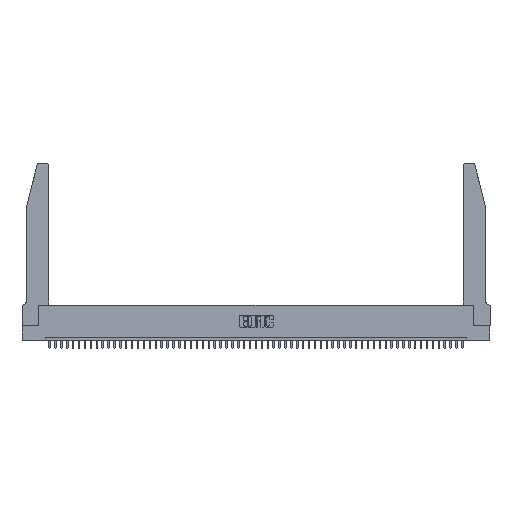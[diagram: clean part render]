
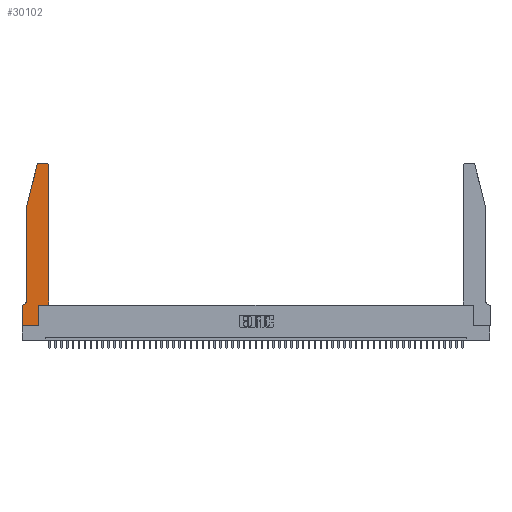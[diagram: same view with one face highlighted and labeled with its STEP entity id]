
A CAD part, top view. The second image highlights one B-rep face of the part: STEP entity #30102.
In plain terms, the highlighted planar face has unit normal (0, 0, 1).
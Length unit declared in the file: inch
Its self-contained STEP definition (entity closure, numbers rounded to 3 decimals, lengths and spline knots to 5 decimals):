
#16 = ORIENTED_EDGE ( 'NONE', *, *, #2910, .T. ) ;
#174 = VERTEX_POINT ( 'NONE', #38158 ) ;
#950 = CIRCLE ( 'NONE', #13804, 0.03 ) ;
#1086 = ORIENTED_EDGE ( 'NONE', *, *, #50567, .T. ) ;
#1452 = CARTESIAN_POINT ( 'NONE',  ( 0.0755, 0.42, 0.37 ) ) ;
#2910 = EDGE_CURVE ( 'NONE', #40060, #28558, #23130, .T. ) ;
#2999 = DIRECTION ( 'NONE',  ( -1., 0., 0. ) ) ;
#3497 = DIRECTION ( 'NONE',  ( -0.239, -0.971, 0. ) ) ;
#4057 = CARTESIAN_POINT ( 'NONE',  ( 0.0755, 2., 0.37 ) ) ;
#4463 = LINE ( 'NONE', #9818, #31969 ) ;
#4713 = CARTESIAN_POINT ( 'NONE',  ( 0.25487, 2.72718, 0.37 ) ) ;
#5218 = CARTESIAN_POINT ( 'NONE',  ( 0.2865, 0.35, 0.37 ) ) ;
#5558 = EDGE_CURVE ( 'NONE', #18067, #16991, #46507, .T. ) ;
#5904 = LINE ( 'NONE', #52612, #53746 ) ;
#6494 = EDGE_CURVE ( 'NONE', #16991, #28098, #20260, .T. ) ;
#6971 = CARTESIAN_POINT ( 'NONE',  ( 0.0755, 0.35, 0.37 ) ) ;
#7023 = CARTESIAN_POINT ( 'NONE',  ( 0.284, 2.72, 0.37 ) ) ;
#7077 = DIRECTION ( 'NONE',  ( 1., 0., 0. ) ) ;
#8402 = CARTESIAN_POINT ( 'NONE',  ( 0., 0., 0.37 ) ) ;
#9818 = CARTESIAN_POINT ( 'NONE',  ( 0., 0., 0.37 ) ) ;
#10351 = CARTESIAN_POINT ( 'NONE',  ( 0.0755, 2., 0.37 ) ) ;
#11780 = VECTOR ( 'NONE', #2999, 39.37008 ) ;
#13215 = ORIENTED_EDGE ( 'NONE', *, *, #16673, .T. ) ;
#13804 = AXIS2_PLACEMENT_3D ( 'NONE', #43182, #18163, #30705 ) ;
#14008 = CARTESIAN_POINT ( 'NONE',  ( 0.284, 2.75, 0.37 ) ) ;
#14403 = ORIENTED_EDGE ( 'NONE', *, *, #17126, .T. ) ;
#14758 = CARTESIAN_POINT ( 'NONE',  ( 0.2865, 0.35, 0.37 ) ) ;
#15021 = DIRECTION ( 'NONE',  ( 0., 0., 1. ) ) ;
#15152 = DIRECTION ( 'NONE',  ( 0., 1., 0. ) ) ;
#15255 = CIRCLE ( 'NONE', #50431, 0.03 ) ;
#15518 = ORIENTED_EDGE ( 'NONE', *, *, #6494, .T. ) ;
#15638 = LINE ( 'NONE', #10351, #32529 ) ;
#15873 = ORIENTED_EDGE ( 'NONE', *, *, #5558, .T. ) ;
#16673 = EDGE_CURVE ( 'NONE', #34504, #174, #27678, .T. ) ;
#16991 = VERTEX_POINT ( 'NONE', #47603 ) ;
#17126 = EDGE_CURVE ( 'NONE', #28558, #34760, #4463, .T. ) ;
#17492 = ORIENTED_EDGE ( 'NONE', *, *, #36888, .T. ) ;
#17604 = VERTEX_POINT ( 'NONE', #51350 ) ;
#17742 = VERTEX_POINT ( 'NONE', #1452 ) ;
#17842 = CARTESIAN_POINT ( 'NONE',  ( 0., 0.35, 0.37 ) ) ;
#18067 = VERTEX_POINT ( 'NONE', #5218 ) ;
#18163 = DIRECTION ( 'NONE',  ( 0., 0., 1. ) ) ;
#19186 = FACE_OUTER_BOUND ( 'NONE', #41227, .T. ) ;
#20111 = DIRECTION ( 'NONE',  ( -1., 0., 0. ) ) ;
#20260 = LINE ( 'NONE', #21286, #35879 ) ;
#20786 = VERTEX_POINT ( 'NONE', #26164 ) ;
#21286 = CARTESIAN_POINT ( 'NONE',  ( 0.4505, 0.35, 0.37 ) ) ;
#23130 = LINE ( 'NONE', #6971, #32956 ) ;
#23139 = DIRECTION ( 'NONE',  ( 0., -1., 0. ) ) ;
#23240 = DIRECTION ( 'NONE',  ( 1., 0., 0. ) ) ;
#25009 = EDGE_CURVE ( 'NONE', #28098, #20786, #950, .T. ) ;
#25452 = LINE ( 'NONE', #44605, #11780 ) ;
#26164 = CARTESIAN_POINT ( 'NONE',  ( 0.4205, 2.75, 0.37 ) ) ;
#26888 = AXIS2_PLACEMENT_3D ( 'NONE', #52086, #15021, #40216 ) ;
#26950 = EDGE_CURVE ( 'NONE', #17742, #40060, #48659, .T. ) ;
#27076 = ORIENTED_EDGE ( 'NONE', *, *, #30351, .T. ) ;
#27678 = LINE ( 'NONE', #4057, #43295 ) ;
#27837 = DIRECTION ( 'NONE',  ( 1., 0., 0. ) ) ;
#28098 = VERTEX_POINT ( 'NONE', #28202 ) ;
#28202 = CARTESIAN_POINT ( 'NONE',  ( 0.4505, 2.72, 0.37 ) ) ;
#28558 = VERTEX_POINT ( 'NONE', #17842 ) ;
#30102 = ADVANCED_FACE ( 'NONE', ( #19186 ), #40026, .T. ) ;
#30351 = EDGE_CURVE ( 'NONE', #46206, #34504, #15255, .T. ) ;
#30705 = DIRECTION ( 'NONE',  ( 1., 0., 0. ) ) ;
#31969 = VECTOR ( 'NONE', #23139, 39.37008 ) ;
#32529 = VECTOR ( 'NONE', #52026, 39.37008 ) ;
#32691 = EDGE_CURVE ( 'NONE', #20786, #46206, #25452, .T. ) ;
#32853 = CARTESIAN_POINT ( 'NONE',  ( 0.0055, 0.35, 0.37 ) ) ;
#32956 = VECTOR ( 'NONE', #40247, 39.37008 ) ;
#34504 = VERTEX_POINT ( 'NONE', #4713 ) ;
#34760 = VERTEX_POINT ( 'NONE', #8402 ) ;
#35879 = VECTOR ( 'NONE', #50223, 39.37008 ) ;
#36888 = EDGE_CURVE ( 'NONE', #34760, #17604, #5904, .T. ) ;
#37429 = ORIENTED_EDGE ( 'NONE', *, *, #50571, .T. ) ;
#38158 = CARTESIAN_POINT ( 'NONE',  ( 0.0755, 2., 0.37 ) ) ;
#40026 = PLANE ( 'NONE',  #26888 ) ;
#40060 = VERTEX_POINT ( 'NONE', #32853 ) ;
#40216 = DIRECTION ( 'NONE',  ( 1., 0., 0. ) ) ;
#40247 = DIRECTION ( 'NONE',  ( -1., 0., 0. ) ) ;
#41227 = EDGE_LOOP ( 'NONE', ( #47808, #27076, #13215, #37429, #43111, #16, #14403, #17492, #1086, #15873, #15518, #52195 ) ) ;
#41975 = VECTOR ( 'NONE', #23240, 39.37008 ) ;
#42998 = VECTOR ( 'NONE', #15152, 39.37008 ) ;
#43111 = ORIENTED_EDGE ( 'NONE', *, *, #26950, .T. ) ;
#43182 = CARTESIAN_POINT ( 'NONE',  ( 0.4205, 2.72, 0.37 ) ) ;
#43295 = VECTOR ( 'NONE', #3497, 39.37008 ) ;
#44106 = CARTESIAN_POINT ( 'NONE',  ( 0.4505, 0.35, 0.37 ) ) ;
#44605 = CARTESIAN_POINT ( 'NONE',  ( 0.2605, 2.75, 0.37 ) ) ;
#45716 = CARTESIAN_POINT ( 'NONE',  ( 0.0055, 0.42, 0.37 ) ) ;
#46206 = VERTEX_POINT ( 'NONE', #14008 ) ;
#46507 = LINE ( 'NONE', #44106, #41975 ) ;
#47603 = CARTESIAN_POINT ( 'NONE',  ( 0.4505, 0.35, 0.37 ) ) ;
#47808 = ORIENTED_EDGE ( 'NONE', *, *, #32691, .T. ) ;
#48659 = CIRCLE ( 'NONE', #52426, 0.07 ) ;
#48914 = DIRECTION ( 'NONE',  ( 0., 0., 1. ) ) ;
#50223 = DIRECTION ( 'NONE',  ( 0., 1., 0. ) ) ;
#50431 = AXIS2_PLACEMENT_3D ( 'NONE', #7023, #48914, #27837 ) ;
#50567 = EDGE_CURVE ( 'NONE', #17604, #18067, #53529, .T. ) ;
#50571 = EDGE_CURVE ( 'NONE', #174, #17742, #15638, .T. ) ;
#51350 = CARTESIAN_POINT ( 'NONE',  ( 0.2865, 0., 0.37 ) ) ;
#52026 = DIRECTION ( 'NONE',  ( 0., -1., 0. ) ) ;
#52086 = CARTESIAN_POINT ( 'NONE',  ( 0., 0.35, 0.37 ) ) ;
#52195 = ORIENTED_EDGE ( 'NONE', *, *, #25009, .T. ) ;
#52426 = AXIS2_PLACEMENT_3D ( 'NONE', #45716, #53939, #20111 ) ;
#52612 = CARTESIAN_POINT ( 'NONE',  ( 0., 0., 0.37 ) ) ;
#53529 = LINE ( 'NONE', #14758, #42998 ) ;
#53746 = VECTOR ( 'NONE', #7077, 39.37008 ) ;
#53939 = DIRECTION ( 'NONE',  ( 0., 0., -1. ) ) ;
